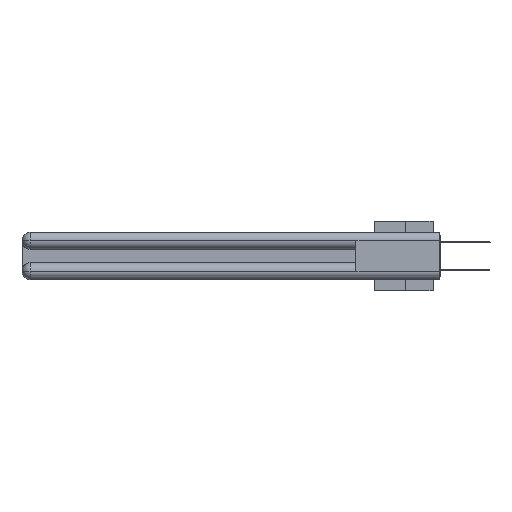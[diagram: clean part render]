
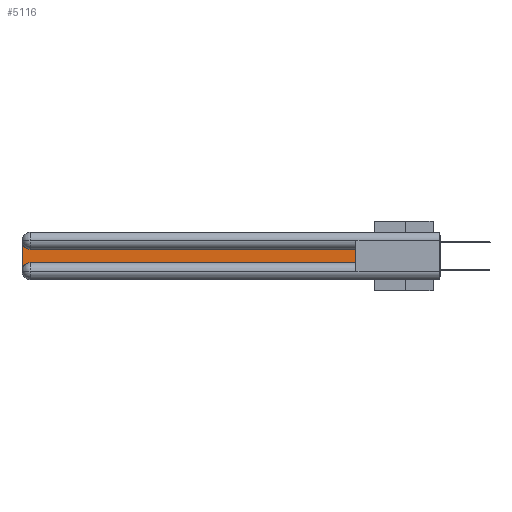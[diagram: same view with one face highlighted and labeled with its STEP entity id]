
A CAD part, left-side view. The second image highlights one B-rep face of the part: STEP entity #5116.
In plain terms, the highlighted planar face has unit normal (-1, 0, 0).
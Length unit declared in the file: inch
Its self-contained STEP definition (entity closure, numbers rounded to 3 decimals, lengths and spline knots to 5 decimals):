
#23 = LINE ( 'NONE', #32828, #6882 ) ;
#74 = ORIENTED_EDGE ( 'NONE', *, *, #3453, .T. ) ;
#851 = CARTESIAN_POINT ( 'NONE',  ( 0.075, 0.6, -0.2175 ) ) ;
#1946 = PLANE ( 'NONE',  #29864 ) ;
#2367 = EDGE_CURVE ( 'NONE', #29575, #18253, #3429, .T. ) ;
#3429 = CIRCLE ( 'NONE', #23479, 0.06 ) ;
#3453 = EDGE_CURVE ( 'NONE', #27468, #29575, #20617, .T. ) ;
#4632 = DIRECTION ( 'NONE',  ( 1., 0., 0. ) ) ;
#4745 = CARTESIAN_POINT ( 'NONE',  ( 0.075, 3., -0.2775 ) ) ;
#4934 = ORIENTED_EDGE ( 'NONE', *, *, #10254, .T. ) ;
#5116 = ADVANCED_FACE ( 'NONE', ( #26317 ), #1946, .F. ) ;
#5267 = LINE ( 'NONE', #12967, #10870 ) ;
#5709 = AXIS2_PLACEMENT_3D ( 'NONE', #12604, #31443, #34489 ) ;
#6134 = CARTESIAN_POINT ( 'NONE',  ( 0.075, 2.94, -0.1225 ) ) ;
#6826 = CARTESIAN_POINT ( 'NONE',  ( 0.075, 3., -0.2175 ) ) ;
#6882 = VECTOR ( 'NONE', #30128, 39.37008 ) ;
#8380 = EDGE_CURVE ( 'NONE', #18253, #33332, #25399, .T. ) ;
#9093 = EDGE_LOOP ( 'NONE', ( #21337, #4934, #74, #29882, #30733, #13804 ) ) ;
#9153 = EDGE_CURVE ( 'NONE', #24081, #28570, #23, .T. ) ;
#10254 = EDGE_CURVE ( 'NONE', #28570, #27468, #29731, .T. ) ;
#10669 = CARTESIAN_POINT ( 'NONE',  ( 0.075, 0.6, -0.2175 ) ) ;
#10870 = VECTOR ( 'NONE', #18872, 39.37008 ) ;
#11589 = DIRECTION ( 'NONE',  ( 0., -1., 0. ) ) ;
#12604 = CARTESIAN_POINT ( 'NONE',  ( 0.075, 2.94, -0.0625 ) ) ;
#12821 = CARTESIAN_POINT ( 'NONE',  ( 0.075, 2.94, -0.2775 ) ) ;
#12853 = CARTESIAN_POINT ( 'NONE',  ( 0.075, 3., -0.1225 ) ) ;
#12967 = CARTESIAN_POINT ( 'NONE',  ( 0.075, 0.6, -0.2175 ) ) ;
#13804 = ORIENTED_EDGE ( 'NONE', *, *, #28370, .T. ) ;
#14228 = CARTESIAN_POINT ( 'NONE',  ( 0.075, 3., -0.0625 ) ) ;
#17905 = CARTESIAN_POINT ( 'NONE',  ( 0.075, 2.94, -0.2175 ) ) ;
#18253 = VERTEX_POINT ( 'NONE', #17905 ) ;
#18872 = DIRECTION ( 'NONE',  ( 0., 0., 1. ) ) ;
#20617 = LINE ( 'NONE', #6826, #31978 ) ;
#20721 = DIRECTION ( 'NONE',  ( 0., 0., -1. ) ) ;
#21337 = ORIENTED_EDGE ( 'NONE', *, *, #9153, .T. ) ;
#23251 = DIRECTION ( 'NONE',  ( 1., 0., 0. ) ) ;
#23479 = AXIS2_PLACEMENT_3D ( 'NONE', #12821, #23251, #20721 ) ;
#23636 = DIRECTION ( 'NONE',  ( 0., 0., -1. ) ) ;
#24081 = VERTEX_POINT ( 'NONE', #30600 ) ;
#24781 = VECTOR ( 'NONE', #11589, 39.37008 ) ;
#25399 = LINE ( 'NONE', #851, #24781 ) ;
#26317 = FACE_OUTER_BOUND ( 'NONE', #9093, .T. ) ;
#27468 = VERTEX_POINT ( 'NONE', #14228 ) ;
#28370 = EDGE_CURVE ( 'NONE', #33332, #24081, #5267, .T. ) ;
#28570 = VERTEX_POINT ( 'NONE', #6134 ) ;
#29575 = VERTEX_POINT ( 'NONE', #4745 ) ;
#29731 = CIRCLE ( 'NONE', #5709, 0.06 ) ;
#29864 = AXIS2_PLACEMENT_3D ( 'NONE', #12853, #4632, #23636 ) ;
#29882 = ORIENTED_EDGE ( 'NONE', *, *, #2367, .T. ) ;
#30128 = DIRECTION ( 'NONE',  ( 0., 1., 0. ) ) ;
#30600 = CARTESIAN_POINT ( 'NONE',  ( 0.075, 0.6, -0.1225 ) ) ;
#30733 = ORIENTED_EDGE ( 'NONE', *, *, #8380, .T. ) ;
#31443 = DIRECTION ( 'NONE',  ( 1., 0., 0. ) ) ;
#31558 = DIRECTION ( 'NONE',  ( 0., 0., -1. ) ) ;
#31978 = VECTOR ( 'NONE', #31558, 39.37008 ) ;
#32828 = CARTESIAN_POINT ( 'NONE',  ( 0.075, 0.6, -0.1225 ) ) ;
#33332 = VERTEX_POINT ( 'NONE', #10669 ) ;
#34489 = DIRECTION ( 'NONE',  ( 0., 0., -1. ) ) ;
